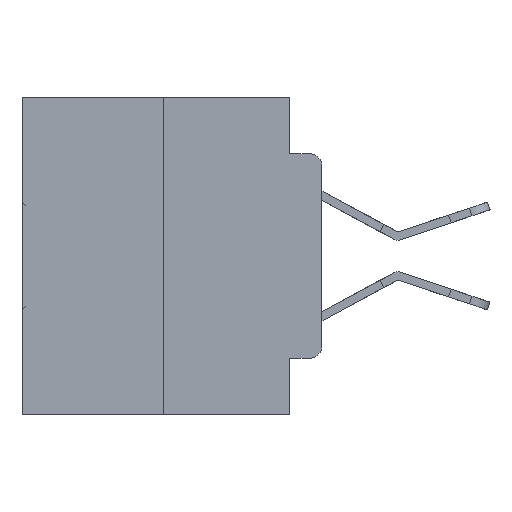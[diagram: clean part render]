
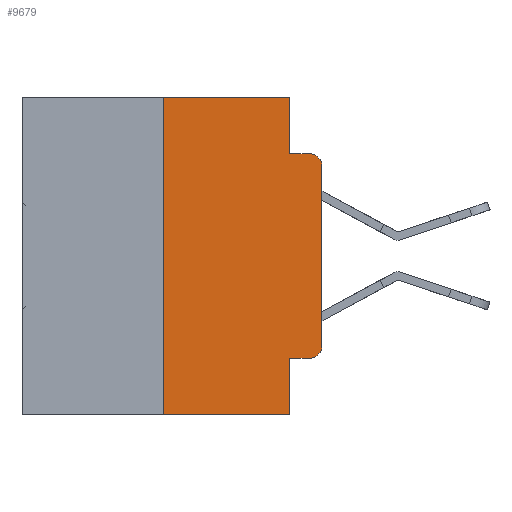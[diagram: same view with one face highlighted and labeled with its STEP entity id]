
A CAD part, left-side view. The second image highlights one B-rep face of the part: STEP entity #9679.
In plain terms, the highlighted planar face has unit normal (-1, 0, 0).
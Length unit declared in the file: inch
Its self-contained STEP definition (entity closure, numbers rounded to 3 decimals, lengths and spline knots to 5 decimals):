
#649 = DIRECTION ( 'NONE',  ( 0., 0., -1. ) ) ;
#673 = LINE ( 'NONE', #12295, #33208 ) ;
#1726 = CARTESIAN_POINT ( 'NONE',  ( 0., 0., -0.3915 ) ) ;
#2409 = DIRECTION ( 'NONE',  ( 0., -1., 0. ) ) ;
#2543 = VERTEX_POINT ( 'NONE', #12481 ) ;
#2717 = VECTOR ( 'NONE', #28232, 39.37008 ) ;
#3914 = CARTESIAN_POINT ( 'NONE',  ( 0., 0.25, 0. ) ) ;
#3951 = AXIS2_PLACEMENT_3D ( 'NONE', #24361, #7843, #7765 ) ;
#4129 = DIRECTION ( 'NONE',  ( 0., 0., -1. ) ) ;
#4152 = ORIENTED_EDGE ( 'NONE', *, *, #25823, .T. ) ;
#4455 = CARTESIAN_POINT ( 'NONE',  ( 0., 0.02, -0.3915 ) ) ;
#5153 = CARTESIAN_POINT ( 'NONE',  ( 0., 0.051, -0.0885 ) ) ;
#5564 = AXIS2_PLACEMENT_3D ( 'NONE', #4455, #22592, #7119 ) ;
#6173 = CARTESIAN_POINT ( 'NONE',  ( 0., 0., 0. ) ) ;
#6224 = DIRECTION ( 'NONE',  ( 0., 0., 1. ) ) ;
#6466 = EDGE_CURVE ( 'NONE', #22455, #2543, #7816, .T. ) ;
#6544 = VERTEX_POINT ( 'NONE', #9907 ) ;
#6599 = DIRECTION ( 'NONE',  ( 0., 0., 1. ) ) ;
#6812 = EDGE_LOOP ( 'NONE', ( #33045, #32894, #26418, #21345, #31892, #26824, #8894, #28411, #4152, #11352 ) ) ;
#7119 = DIRECTION ( 'NONE',  ( 0., 0., -1. ) ) ;
#7765 = DIRECTION ( 'NONE',  ( 0., 0., -1. ) ) ;
#7779 = CARTESIAN_POINT ( 'NONE',  ( 0., 0.051, -0.4115 ) ) ;
#7816 = CIRCLE ( 'NONE', #3951, 0.02 ) ;
#7843 = DIRECTION ( 'NONE',  ( -1., 0., 0. ) ) ;
#8721 = EDGE_CURVE ( 'NONE', #15994, #22455, #17850, .T. ) ;
#8894 = ORIENTED_EDGE ( 'NONE', *, *, #17376, .T. ) ;
#9679 = ADVANCED_FACE ( 'NONE', ( #24480 ), #24001, .F. ) ;
#9818 = LINE ( 'NONE', #5153, #2717 ) ;
#9907 = CARTESIAN_POINT ( 'NONE',  ( 0., 0.02, -0.4115 ) ) ;
#10256 = CARTESIAN_POINT ( 'NONE',  ( 0., 0.473, -0.5 ) ) ;
#10418 = DIRECTION ( 'NONE',  ( 0., 0., -1. ) ) ;
#10502 = EDGE_CURVE ( 'NONE', #32054, #12342, #673, .T. ) ;
#11352 = ORIENTED_EDGE ( 'NONE', *, *, #27513, .T. ) ;
#12175 = VECTOR ( 'NONE', #10418, 39.37008 ) ;
#12295 = CARTESIAN_POINT ( 'NONE',  ( 0., 0.051, 0. ) ) ;
#12342 = VERTEX_POINT ( 'NONE', #31301 ) ;
#12481 = CARTESIAN_POINT ( 'NONE',  ( 0., 0.02, -0.0885 ) ) ;
#12552 = VERTEX_POINT ( 'NONE', #29683 ) ;
#13045 = CARTESIAN_POINT ( 'NONE',  ( 0., 0.051, 0. ) ) ;
#13136 = LINE ( 'NONE', #10256, #19099 ) ;
#14087 = VECTOR ( 'NONE', #2409, 39.37008 ) ;
#14898 = LINE ( 'NONE', #7779, #14087 ) ;
#15283 = LINE ( 'NONE', #3914, #21198 ) ;
#15430 = VERTEX_POINT ( 'NONE', #30311 ) ;
#15994 = VERTEX_POINT ( 'NONE', #1726 ) ;
#16478 = DIRECTION ( 'NONE',  ( 1., 0., 0. ) ) ;
#17376 = EDGE_CURVE ( 'NONE', #15430, #21886, #13136, .T. ) ;
#17442 = EDGE_CURVE ( 'NONE', #12342, #2543, #9818, .T. ) ;
#17850 = LINE ( 'NONE', #6173, #29576 ) ;
#18057 = DIRECTION ( 'NONE',  ( 0., -1., 0. ) ) ;
#19099 = VECTOR ( 'NONE', #28024, 39.37008 ) ;
#19122 = EDGE_CURVE ( 'NONE', #24148, #21886, #31469, .T. ) ;
#20792 = EDGE_CURVE ( 'NONE', #15430, #12552, #15283, .T. ) ;
#21198 = VECTOR ( 'NONE', #6599, 39.37008 ) ;
#21249 = CARTESIAN_POINT ( 'NONE',  ( 0., 0.051, -0.5 ) ) ;
#21345 = ORIENTED_EDGE ( 'NONE', *, *, #10502, .F. ) ;
#21444 = CARTESIAN_POINT ( 'NONE',  ( 0., 0.473, 0. ) ) ;
#21886 = VERTEX_POINT ( 'NONE', #21249 ) ;
#22455 = VERTEX_POINT ( 'NONE', #30815 ) ;
#22592 = DIRECTION ( 'NONE',  ( -1., 0., 0. ) ) ;
#24001 = PLANE ( 'NONE',  #32493 ) ;
#24078 = LINE ( 'NONE', #33001, #29895 ) ;
#24148 = VERTEX_POINT ( 'NONE', #30890 ) ;
#24361 = CARTESIAN_POINT ( 'NONE',  ( 0., 0.02, -0.1085 ) ) ;
#24480 = FACE_OUTER_BOUND ( 'NONE', #6812, .T. ) ;
#24659 = CIRCLE ( 'NONE', #5564, 0.02 ) ;
#25638 = CARTESIAN_POINT ( 'NONE',  ( 0., 0.051, 0. ) ) ;
#25823 = EDGE_CURVE ( 'NONE', #24148, #6544, #14898, .T. ) ;
#26418 = ORIENTED_EDGE ( 'NONE', *, *, #17442, .F. ) ;
#26824 = ORIENTED_EDGE ( 'NONE', *, *, #20792, .F. ) ;
#27513 = EDGE_CURVE ( 'NONE', #6544, #15994, #24659, .T. ) ;
#28024 = DIRECTION ( 'NONE',  ( 0., -1., 0. ) ) ;
#28232 = DIRECTION ( 'NONE',  ( 0., -1., 0. ) ) ;
#28411 = ORIENTED_EDGE ( 'NONE', *, *, #19122, .F. ) ;
#29576 = VECTOR ( 'NONE', #6224, 39.37008 ) ;
#29683 = CARTESIAN_POINT ( 'NONE',  ( 0., 0.25, 0. ) ) ;
#29895 = VECTOR ( 'NONE', #18057, 39.37008 ) ;
#30221 = EDGE_CURVE ( 'NONE', #12552, #32054, #24078, .T. ) ;
#30311 = CARTESIAN_POINT ( 'NONE',  ( 0., 0.25, -0.5 ) ) ;
#30815 = CARTESIAN_POINT ( 'NONE',  ( 0., 0., -0.1085 ) ) ;
#30890 = CARTESIAN_POINT ( 'NONE',  ( 0., 0.051, -0.4115 ) ) ;
#31301 = CARTESIAN_POINT ( 'NONE',  ( 0., 0.051, -0.0885 ) ) ;
#31469 = LINE ( 'NONE', #25638, #12175 ) ;
#31892 = ORIENTED_EDGE ( 'NONE', *, *, #30221, .F. ) ;
#32054 = VERTEX_POINT ( 'NONE', #13045 ) ;
#32493 = AXIS2_PLACEMENT_3D ( 'NONE', #21444, #16478, #649 ) ;
#32894 = ORIENTED_EDGE ( 'NONE', *, *, #6466, .T. ) ;
#33001 = CARTESIAN_POINT ( 'NONE',  ( 0., 0.473, 0. ) ) ;
#33045 = ORIENTED_EDGE ( 'NONE', *, *, #8721, .T. ) ;
#33208 = VECTOR ( 'NONE', #4129, 39.37008 ) ;
